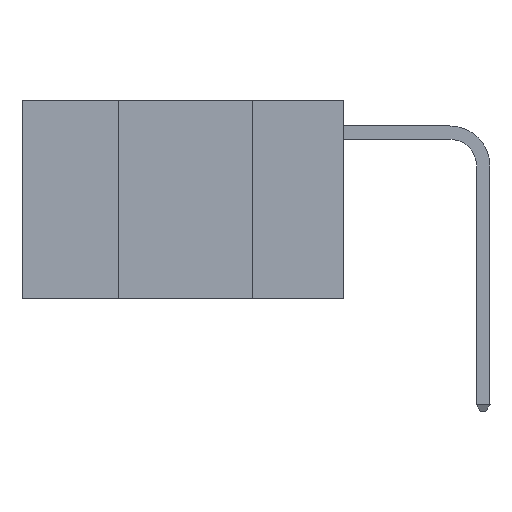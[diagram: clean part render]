
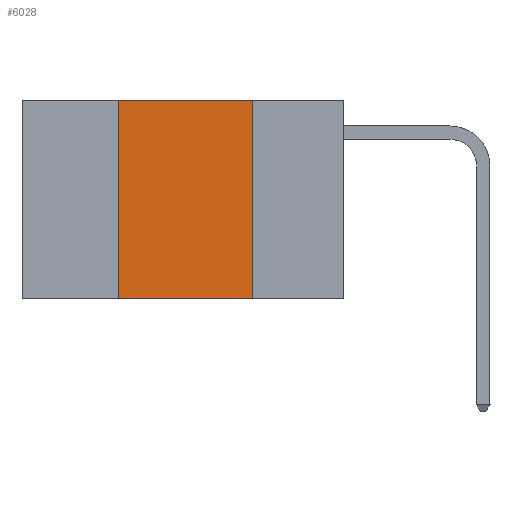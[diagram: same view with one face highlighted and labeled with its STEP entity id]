
A CAD part, left-side view. The second image highlights one B-rep face of the part: STEP entity #6028.
In plain terms, the highlighted planar face has unit normal (-1, 0, 0).
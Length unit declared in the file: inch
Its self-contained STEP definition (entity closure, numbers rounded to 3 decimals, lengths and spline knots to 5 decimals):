
#280 = ORIENTED_EDGE ( 'NONE', *, *, #22641, .F. ) ;
#328 = ORIENTED_EDGE ( 'NONE', *, *, #874, .F. ) ;
#430 = CARTESIAN_POINT ( 'NONE',  ( 0., 0.6, -0.37 ) ) ;
#874 = EDGE_CURVE ( 'NONE', #24194, #4665, #7042, .T. ) ;
#1938 = EDGE_LOOP ( 'NONE', ( #280, #328, #27675, #12901 ) ) ;
#2193 = VECTOR ( 'NONE', #17819, 39.37008 ) ;
#2598 = DIRECTION ( 'NONE',  ( 0., -1., 0. ) ) ;
#2874 = CARTESIAN_POINT ( 'NONE',  ( 0., 0.6, 0. ) ) ;
#3070 = LINE ( 'NONE', #20409, #20779 ) ;
#4595 = CARTESIAN_POINT ( 'NONE',  ( 0., 0.17, -0.37 ) ) ;
#4665 = VERTEX_POINT ( 'NONE', #23948 ) ;
#5420 = AXIS2_PLACEMENT_3D ( 'NONE', #25062, #20695, #26891 ) ;
#6028 = ADVANCED_FACE ( 'NONE', ( #22787 ), #7815, .F. ) ;
#7042 = LINE ( 'NONE', #2874, #9860 ) ;
#7815 = PLANE ( 'NONE',  #5420 ) ;
#9860 = VECTOR ( 'NONE', #2598, 39.37008 ) ;
#11082 = CARTESIAN_POINT ( 'NONE',  ( 0., 0.17, 0. ) ) ;
#11177 = DIRECTION ( 'NONE',  ( 0., -1., 0. ) ) ;
#11372 = VECTOR ( 'NONE', #11177, 39.37008 ) ;
#12901 = ORIENTED_EDGE ( 'NONE', *, *, #20395, .T. ) ;
#17819 = DIRECTION ( 'NONE',  ( 0., 0., -1. ) ) ;
#18735 = EDGE_CURVE ( 'NONE', #18910, #24194, #3070, .T. ) ;
#18910 = VERTEX_POINT ( 'NONE', #24292 ) ;
#19598 = LINE ( 'NONE', #430, #11372 ) ;
#19779 = LINE ( 'NONE', #11082, #2193 ) ;
#20395 = EDGE_CURVE ( 'NONE', #18910, #26541, #19598, .T. ) ;
#20409 = CARTESIAN_POINT ( 'NONE',  ( 0., 0.42, 0. ) ) ;
#20695 = DIRECTION ( 'NONE',  ( 1., 0., 0. ) ) ;
#20779 = VECTOR ( 'NONE', #22370, 39.37008 ) ;
#22370 = DIRECTION ( 'NONE',  ( 0., 0., 1. ) ) ;
#22641 = EDGE_CURVE ( 'NONE', #4665, #26541, #19779, .T. ) ;
#22787 = FACE_OUTER_BOUND ( 'NONE', #1938, .T. ) ;
#23948 = CARTESIAN_POINT ( 'NONE',  ( 0., 0.17, 0. ) ) ;
#24194 = VERTEX_POINT ( 'NONE', #24841 ) ;
#24292 = CARTESIAN_POINT ( 'NONE',  ( 0., 0.42, -0.37 ) ) ;
#24841 = CARTESIAN_POINT ( 'NONE',  ( 0., 0.42, 0. ) ) ;
#25062 = CARTESIAN_POINT ( 'NONE',  ( 0., 0.6, 0. ) ) ;
#26541 = VERTEX_POINT ( 'NONE', #4595 ) ;
#26891 = DIRECTION ( 'NONE',  ( 0., 0., -1. ) ) ;
#27675 = ORIENTED_EDGE ( 'NONE', *, *, #18735, .F. ) ;
